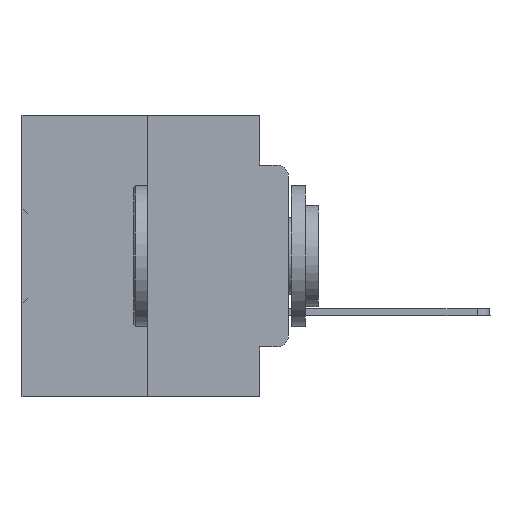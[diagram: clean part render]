
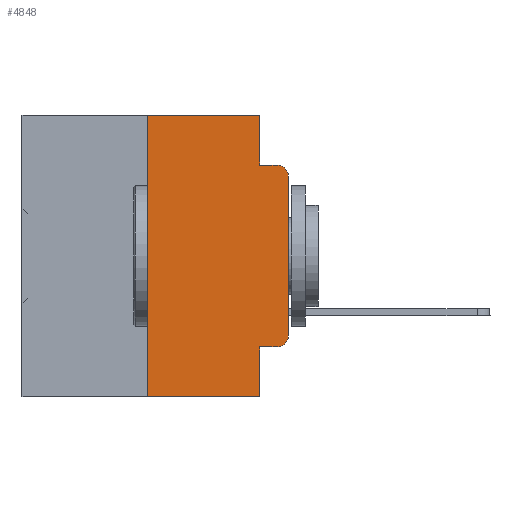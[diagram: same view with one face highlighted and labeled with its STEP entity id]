
A CAD part, left-side view. The second image highlights one B-rep face of the part: STEP entity #4848.
In plain terms, the highlighted planar face has unit normal (-1, 0, 0).
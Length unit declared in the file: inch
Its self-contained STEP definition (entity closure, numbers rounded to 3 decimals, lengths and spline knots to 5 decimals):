
#84 = EDGE_CURVE ( 'NONE', #5191, #14613, #7481, .T. ) ;
#133 = DIRECTION ( 'NONE',  ( 0., 0., 1. ) ) ;
#1658 = FACE_OUTER_BOUND ( 'NONE', #26113, .T. ) ;
#1784 = LINE ( 'NONE', #35018, #36881 ) ;
#1819 = DIRECTION ( 'NONE',  ( 0., -1., 0. ) ) ;
#2142 = ORIENTED_EDGE ( 'NONE', *, *, #8247, .F. ) ;
#3396 = DIRECTION ( 'NONE',  ( 0., 0., -1. ) ) ;
#4013 = DIRECTION ( 'NONE',  ( 0., 0., 1. ) ) ;
#4848 = ADVANCED_FACE ( 'NONE', ( #1658 ), #13562, .F. ) ;
#4877 = ORIENTED_EDGE ( 'NONE', *, *, #23625, .T. ) ;
#5191 = VERTEX_POINT ( 'NONE', #37603 ) ;
#5384 = LINE ( 'NONE', #12395, #13624 ) ;
#5855 = VERTEX_POINT ( 'NONE', #29504 ) ;
#7207 = EDGE_CURVE ( 'NONE', #5855, #7314, #1784, .T. ) ;
#7314 = VERTEX_POINT ( 'NONE', #29907 ) ;
#7481 = LINE ( 'NONE', #26100, #30707 ) ;
#7605 = CIRCLE ( 'NONE', #9976, 0.02 ) ;
#8247 = EDGE_CURVE ( 'NONE', #5855, #25000, #24996, .T. ) ;
#8680 = CARTESIAN_POINT ( 'NONE',  ( 0., 0., 0. ) ) ;
#8733 = ORIENTED_EDGE ( 'NONE', *, *, #18841, .T. ) ;
#8837 = VECTOR ( 'NONE', #4013, 39.37008 ) ;
#9310 = VECTOR ( 'NONE', #25663, 39.37008 ) ;
#9804 = ORIENTED_EDGE ( 'NONE', *, *, #30783, .F. ) ;
#9976 = AXIS2_PLACEMENT_3D ( 'NONE', #27435, #22104, #16174 ) ;
#10955 = CARTESIAN_POINT ( 'NONE',  ( 0., 0.25, -0.5 ) ) ;
#12395 = CARTESIAN_POINT ( 'NONE',  ( 0., 0.473, 0. ) ) ;
#12458 = VERTEX_POINT ( 'NONE', #22583 ) ;
#13348 = CARTESIAN_POINT ( 'NONE',  ( 0., 0.25, 0. ) ) ;
#13562 = PLANE ( 'NONE',  #28430 ) ;
#13624 = VECTOR ( 'NONE', #30306, 39.37008 ) ;
#14580 = ORIENTED_EDGE ( 'NONE', *, *, #18398, .T. ) ;
#14613 = VERTEX_POINT ( 'NONE', #24933 ) ;
#15046 = CARTESIAN_POINT ( 'NONE',  ( 0., 0.02, -0.3915 ) ) ;
#15943 = ORIENTED_EDGE ( 'NONE', *, *, #35449, .T. ) ;
#16174 = DIRECTION ( 'NONE',  ( 0., 0., -1. ) ) ;
#17090 = LINE ( 'NONE', #31279, #9310 ) ;
#17136 = ORIENTED_EDGE ( 'NONE', *, *, #35621, .F. ) ;
#17601 = DIRECTION ( 'NONE',  ( 0., -1., 0. ) ) ;
#18398 = EDGE_CURVE ( 'NONE', #7314, #27472, #22566, .T. ) ;
#18841 = EDGE_CURVE ( 'NONE', #23070, #25000, #17090, .T. ) ;
#18910 = LINE ( 'NONE', #13348, #8837 ) ;
#20483 = LINE ( 'NONE', #8680, #22727 ) ;
#22104 = DIRECTION ( 'NONE',  ( -1., 0., 0. ) ) ;
#22566 = CIRCLE ( 'NONE', #23025, 0.02 ) ;
#22583 = CARTESIAN_POINT ( 'NONE',  ( 0., 0.25, 0. ) ) ;
#22727 = VECTOR ( 'NONE', #133, 39.37008 ) ;
#23025 = AXIS2_PLACEMENT_3D ( 'NONE', #15046, #26601, #3396 ) ;
#23038 = DIRECTION ( 'NONE',  ( 0., 0., -1. ) ) ;
#23070 = VERTEX_POINT ( 'NONE', #10955 ) ;
#23625 = EDGE_CURVE ( 'NONE', #32927, #35690, #7605, .T. ) ;
#24691 = EDGE_CURVE ( 'NONE', #14613, #35690, #37400, .T. ) ;
#24933 = CARTESIAN_POINT ( 'NONE',  ( 0., 0.051, -0.0885 ) ) ;
#24996 = LINE ( 'NONE', #28550, #26287 ) ;
#25000 = VERTEX_POINT ( 'NONE', #26014 ) ;
#25028 = CARTESIAN_POINT ( 'NONE',  ( 0., 0.051, -0.0885 ) ) ;
#25393 = DIRECTION ( 'NONE',  ( 0., 0., -1. ) ) ;
#25663 = DIRECTION ( 'NONE',  ( 0., -1., 0. ) ) ;
#26014 = CARTESIAN_POINT ( 'NONE',  ( 0., 0.051, -0.5 ) ) ;
#26100 = CARTESIAN_POINT ( 'NONE',  ( 0., 0.051, 0. ) ) ;
#26113 = EDGE_LOOP ( 'NONE', ( #15943, #4877, #29573, #29569, #17136, #9804, #8733, #2142, #29126, #14580 ) ) ;
#26287 = VECTOR ( 'NONE', #25393, 39.37008 ) ;
#26601 = DIRECTION ( 'NONE',  ( -1., 0., 0. ) ) ;
#27435 = CARTESIAN_POINT ( 'NONE',  ( 0., 0.02, -0.1085 ) ) ;
#27472 = VERTEX_POINT ( 'NONE', #29844 ) ;
#28430 = AXIS2_PLACEMENT_3D ( 'NONE', #30731, #30859, #36348 ) ;
#28550 = CARTESIAN_POINT ( 'NONE',  ( 0., 0.051, 0. ) ) ;
#29126 = ORIENTED_EDGE ( 'NONE', *, *, #7207, .T. ) ;
#29504 = CARTESIAN_POINT ( 'NONE',  ( 0., 0.051, -0.4115 ) ) ;
#29569 = ORIENTED_EDGE ( 'NONE', *, *, #84, .F. ) ;
#29573 = ORIENTED_EDGE ( 'NONE', *, *, #24691, .F. ) ;
#29643 = VECTOR ( 'NONE', #1819, 39.37008 ) ;
#29844 = CARTESIAN_POINT ( 'NONE',  ( 0., 0., -0.3915 ) ) ;
#29907 = CARTESIAN_POINT ( 'NONE',  ( 0., 0.02, -0.4115 ) ) ;
#29926 = CARTESIAN_POINT ( 'NONE',  ( 0., 0.02, -0.0885 ) ) ;
#30306 = DIRECTION ( 'NONE',  ( 0., -1., 0. ) ) ;
#30707 = VECTOR ( 'NONE', #23038, 39.37008 ) ;
#30731 = CARTESIAN_POINT ( 'NONE',  ( 0., 0.473, 0. ) ) ;
#30783 = EDGE_CURVE ( 'NONE', #23070, #12458, #18910, .T. ) ;
#30859 = DIRECTION ( 'NONE',  ( 1., 0., 0. ) ) ;
#31279 = CARTESIAN_POINT ( 'NONE',  ( 0., 0.473, -0.5 ) ) ;
#32927 = VERTEX_POINT ( 'NONE', #36293 ) ;
#35018 = CARTESIAN_POINT ( 'NONE',  ( 0., 0.051, -0.4115 ) ) ;
#35449 = EDGE_CURVE ( 'NONE', #27472, #32927, #20483, .T. ) ;
#35621 = EDGE_CURVE ( 'NONE', #12458, #5191, #5384, .T. ) ;
#35690 = VERTEX_POINT ( 'NONE', #29926 ) ;
#36293 = CARTESIAN_POINT ( 'NONE',  ( 0., 0., -0.1085 ) ) ;
#36348 = DIRECTION ( 'NONE',  ( 0., 0., -1. ) ) ;
#36881 = VECTOR ( 'NONE', #17601, 39.37008 ) ;
#37400 = LINE ( 'NONE', #25028, #29643 ) ;
#37603 = CARTESIAN_POINT ( 'NONE',  ( 0., 0.051, 0. ) ) ;
